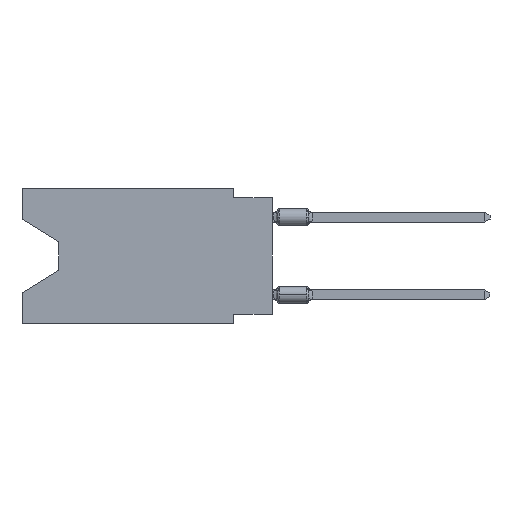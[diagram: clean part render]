
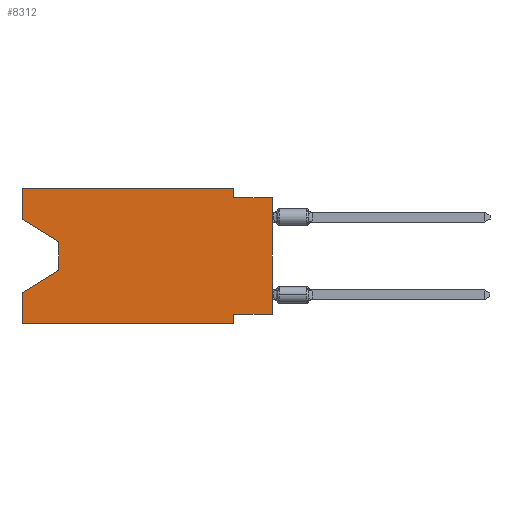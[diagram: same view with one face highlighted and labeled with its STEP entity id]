
A CAD part, left-side view. The second image highlights one B-rep face of the part: STEP entity #8312.
In plain terms, the highlighted planar face has unit normal (-1, 0, 0).
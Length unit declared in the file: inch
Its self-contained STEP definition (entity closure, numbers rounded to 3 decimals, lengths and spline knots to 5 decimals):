
#78 = CARTESIAN_POINT ( 'NONE',  ( 0., 0.645, 0. ) ) ;
#241 = DIRECTION ( 'NONE',  ( 0., 0., 1. ) ) ;
#408 = CARTESIAN_POINT ( 'NONE',  ( 0., 0., 0. ) ) ;
#601 = CARTESIAN_POINT ( 'NONE',  ( 0., 0.55, -0.138 ) ) ;
#763 = CARTESIAN_POINT ( 'NONE',  ( 0., 0.1, -0.025 ) ) ;
#1009 = VERTEX_POINT ( 'NONE', #2228 ) ;
#1135 = EDGE_CURVE ( 'NONE', #8529, #13644, #6636, .T. ) ;
#1397 = DIRECTION ( 'NONE',  ( 0., 0., 1. ) ) ;
#1416 = VECTOR ( 'NONE', #2563, 39.37008 ) ;
#1903 = LINE ( 'NONE', #5281, #3938 ) ;
#2109 = LINE ( 'NONE', #4392, #8983 ) ;
#2228 = CARTESIAN_POINT ( 'NONE',  ( 0., 0., -0.325 ) ) ;
#2234 = CARTESIAN_POINT ( 'NONE',  ( 0., 0.645, 0. ) ) ;
#2302 = DIRECTION ( 'NONE',  ( 0., -1., 0. ) ) ;
#2563 = DIRECTION ( 'NONE',  ( 0., 0., 1. ) ) ;
#2945 = VECTOR ( 'NONE', #8337, 39.37008 ) ;
#3078 = PLANE ( 'NONE',  #8023 ) ;
#3148 = VERTEX_POINT ( 'NONE', #11390 ) ;
#3150 = DIRECTION ( 'NONE',  ( 0., -1., 0. ) ) ;
#3169 = DIRECTION ( 'NONE',  ( 0., 0., -1. ) ) ;
#3707 = VERTEX_POINT ( 'NONE', #4739 ) ;
#3753 = CARTESIAN_POINT ( 'NONE',  ( 0., 0.1, -0.35 ) ) ;
#3929 = LINE ( 'NONE', #4754, #12620 ) ;
#3930 = EDGE_LOOP ( 'NONE', ( #12561, #12037, #10196, #8055, #7679, #8071, #8786, #6096, #4069, #7708, #5056, #11508 ) ) ;
#3938 = VECTOR ( 'NONE', #3150, 39.37008 ) ;
#3993 = EDGE_CURVE ( 'NONE', #1009, #4228, #2109, .T. ) ;
#4069 = ORIENTED_EDGE ( 'NONE', *, *, #4959, .F. ) ;
#4208 = CARTESIAN_POINT ( 'NONE',  ( 0., 0.645, 0. ) ) ;
#4228 = VERTEX_POINT ( 'NONE', #12153 ) ;
#4273 = EDGE_CURVE ( 'NONE', #8529, #8474, #1903, .T. ) ;
#4392 = CARTESIAN_POINT ( 'NONE',  ( 0., 0., -0.325 ) ) ;
#4594 = DIRECTION ( 'NONE',  ( 0., 0.855, -0.519 ) ) ;
#4739 = CARTESIAN_POINT ( 'NONE',  ( 0., 0.55, -0.212 ) ) ;
#4754 = CARTESIAN_POINT ( 'NONE',  ( 0., 0., -0.025 ) ) ;
#4775 = CARTESIAN_POINT ( 'NONE',  ( 0., 0.645, -0.35 ) ) ;
#4887 = DIRECTION ( 'NONE',  ( 0., -1., 0. ) ) ;
#4959 = EDGE_CURVE ( 'NONE', #12306, #9147, #3929, .T. ) ;
#5056 = ORIENTED_EDGE ( 'NONE', *, *, #10751, .F. ) ;
#5281 = CARTESIAN_POINT ( 'NONE',  ( 0., 0.645, -0.35 ) ) ;
#5386 = VERTEX_POINT ( 'NONE', #12165 ) ;
#5464 = EDGE_CURVE ( 'NONE', #3148, #12306, #12442, .T. ) ;
#5570 = EDGE_CURVE ( 'NONE', #3707, #13644, #10632, .T. ) ;
#5657 = DIRECTION ( 'NONE',  ( 0., 0., -1. ) ) ;
#5812 = VECTOR ( 'NONE', #9459, 39.37008 ) ;
#6096 = ORIENTED_EDGE ( 'NONE', *, *, #7331, .T. ) ;
#6220 = EDGE_CURVE ( 'NONE', #6871, #5386, #10393, .T. ) ;
#6296 = CARTESIAN_POINT ( 'NONE',  ( 0., 0.645, 0. ) ) ;
#6636 = LINE ( 'NONE', #10824, #10542 ) ;
#6795 = VERTEX_POINT ( 'NONE', #2234 ) ;
#6871 = VERTEX_POINT ( 'NONE', #8705 ) ;
#7117 = DIRECTION ( 'NONE',  ( 1., 0., 0. ) ) ;
#7198 = VECTOR ( 'NONE', #2302, 39.37008 ) ;
#7331 = EDGE_CURVE ( 'NONE', #1009, #9147, #13043, .T. ) ;
#7426 = LINE ( 'NONE', #9682, #10653 ) ;
#7679 = ORIENTED_EDGE ( 'NONE', *, *, #4273, .T. ) ;
#7708 = ORIENTED_EDGE ( 'NONE', *, *, #5464, .F. ) ;
#7785 = EDGE_CURVE ( 'NONE', #5386, #3707, #8809, .T. ) ;
#7966 = EDGE_CURVE ( 'NONE', #4228, #8474, #7426, .T. ) ;
#8023 = AXIS2_PLACEMENT_3D ( 'NONE', #6296, #7117, #8483 ) ;
#8055 = ORIENTED_EDGE ( 'NONE', *, *, #1135, .F. ) ;
#8071 = ORIENTED_EDGE ( 'NONE', *, *, #7966, .F. ) ;
#8312 = ADVANCED_FACE ( 'NONE', ( #12429 ), #3078, .F. ) ;
#8337 = DIRECTION ( 'NONE',  ( 0., -0.855, -0.519 ) ) ;
#8407 = VECTOR ( 'NONE', #4594, 39.37008 ) ;
#8474 = VERTEX_POINT ( 'NONE', #3753 ) ;
#8483 = DIRECTION ( 'NONE',  ( 0., 0., -1. ) ) ;
#8529 = VERTEX_POINT ( 'NONE', #4775 ) ;
#8705 = CARTESIAN_POINT ( 'NONE',  ( 0., 0.645, -0.08025 ) ) ;
#8786 = ORIENTED_EDGE ( 'NONE', *, *, #3993, .F. ) ;
#8809 = LINE ( 'NONE', #601, #9114 ) ;
#8983 = VECTOR ( 'NONE', #10506, 39.37008 ) ;
#9114 = VECTOR ( 'NONE', #5657, 39.37008 ) ;
#9147 = VERTEX_POINT ( 'NONE', #13651 ) ;
#9459 = DIRECTION ( 'NONE',  ( 0., 0., -1. ) ) ;
#9523 = LINE ( 'NONE', #78, #7198 ) ;
#9665 = CARTESIAN_POINT ( 'NONE',  ( 0., 0.55, -0.212 ) ) ;
#9682 = CARTESIAN_POINT ( 'NONE',  ( 0., 0.1, -0.35 ) ) ;
#10058 = VECTOR ( 'NONE', #241, 39.37008 ) ;
#10196 = ORIENTED_EDGE ( 'NONE', *, *, #5570, .T. ) ;
#10373 = CARTESIAN_POINT ( 'NONE',  ( 0., 0.645, -0.26975 ) ) ;
#10393 = LINE ( 'NONE', #11500, #2945 ) ;
#10506 = DIRECTION ( 'NONE',  ( 0., 1., 0. ) ) ;
#10542 = VECTOR ( 'NONE', #1397, 39.37008 ) ;
#10632 = LINE ( 'NONE', #9665, #8407 ) ;
#10653 = VECTOR ( 'NONE', #3169, 39.37008 ) ;
#10751 = EDGE_CURVE ( 'NONE', #6795, #3148, #9523, .T. ) ;
#10824 = CARTESIAN_POINT ( 'NONE',  ( 0., 0.645, 0. ) ) ;
#11390 = CARTESIAN_POINT ( 'NONE',  ( 0., 0.1, 0. ) ) ;
#11500 = CARTESIAN_POINT ( 'NONE',  ( 0., 0.645, -0.08025 ) ) ;
#11508 = ORIENTED_EDGE ( 'NONE', *, *, #13349, .F. ) ;
#12037 = ORIENTED_EDGE ( 'NONE', *, *, #7785, .T. ) ;
#12153 = CARTESIAN_POINT ( 'NONE',  ( 0., 0.1, -0.325 ) ) ;
#12165 = CARTESIAN_POINT ( 'NONE',  ( 0., 0.55, -0.138 ) ) ;
#12306 = VERTEX_POINT ( 'NONE', #763 ) ;
#12429 = FACE_OUTER_BOUND ( 'NONE', #3930, .T. ) ;
#12442 = LINE ( 'NONE', #12647, #5812 ) ;
#12561 = ORIENTED_EDGE ( 'NONE', *, *, #6220, .T. ) ;
#12620 = VECTOR ( 'NONE', #4887, 39.37008 ) ;
#12647 = CARTESIAN_POINT ( 'NONE',  ( 0., 0.1, 0. ) ) ;
#13043 = LINE ( 'NONE', #408, #1416 ) ;
#13349 = EDGE_CURVE ( 'NONE', #6871, #6795, #13648, .T. ) ;
#13644 = VERTEX_POINT ( 'NONE', #10373 ) ;
#13648 = LINE ( 'NONE', #4208, #10058 ) ;
#13651 = CARTESIAN_POINT ( 'NONE',  ( 0., 0., -0.025 ) ) ;
